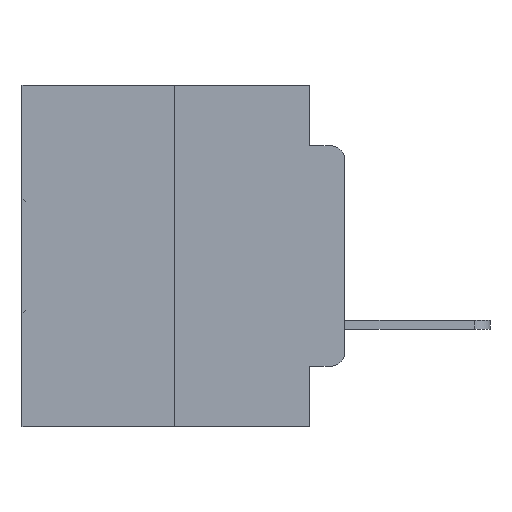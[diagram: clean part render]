
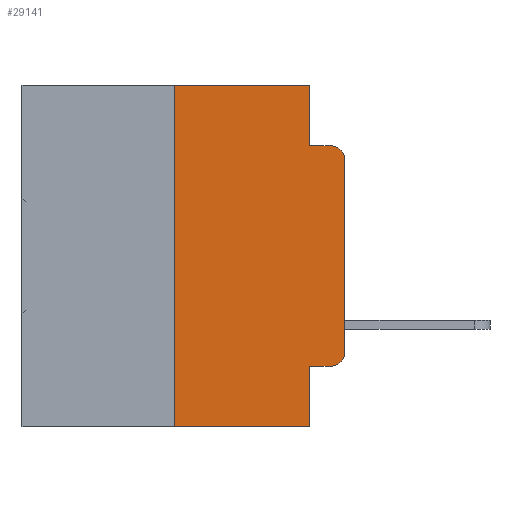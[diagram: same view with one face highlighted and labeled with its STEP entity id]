
A CAD part, left-side view. The second image highlights one B-rep face of the part: STEP entity #29141.
In plain terms, the highlighted planar face has unit normal (-1, 0, 0).
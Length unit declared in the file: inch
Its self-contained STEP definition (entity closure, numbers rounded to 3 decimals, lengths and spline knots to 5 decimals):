
#12 = CARTESIAN_POINT ( 'NONE',  ( 0., 0.25, -0.5 ) ) ;
#432 = EDGE_CURVE ( 'NONE', #4082, #10089, #1228, .T. ) ;
#1228 = CIRCLE ( 'NONE', #27932, 0.02 ) ;
#1529 = AXIS2_PLACEMENT_3D ( 'NONE', #28865, #9449, #2348 ) ;
#2348 = DIRECTION ( 'NONE',  ( 0., 0., -1. ) ) ;
#3346 = DIRECTION ( 'NONE',  ( 0., -1., 0. ) ) ;
#3621 = CARTESIAN_POINT ( 'NONE',  ( 0., 0.051, -0.0885 ) ) ;
#3877 = LINE ( 'NONE', #9337, #23126 ) ;
#4082 = VERTEX_POINT ( 'NONE', #4563 ) ;
#4563 = CARTESIAN_POINT ( 'NONE',  ( 0., 0.02, -0.4115 ) ) ;
#4642 = LINE ( 'NONE', #19260, #14094 ) ;
#4684 = DIRECTION ( 'NONE',  ( 0., 0., -1. ) ) ;
#5099 = ORIENTED_EDGE ( 'NONE', *, *, #18385, .T. ) ;
#5803 = EDGE_CURVE ( 'NONE', #26232, #4082, #29390, .T. ) ;
#7179 = EDGE_CURVE ( 'NONE', #28852, #25640, #28449, .T. ) ;
#8128 = VERTEX_POINT ( 'NONE', #12 ) ;
#8227 = FACE_OUTER_BOUND ( 'NONE', #29650, .T. ) ;
#8229 = DIRECTION ( 'NONE',  ( 0., -1., 0. ) ) ;
#8616 = LINE ( 'NONE', #27436, #13507 ) ;
#8638 = DIRECTION ( 'NONE',  ( 0., 0., -1. ) ) ;
#8962 = VECTOR ( 'NONE', #25877, 39.37008 ) ;
#9337 = CARTESIAN_POINT ( 'NONE',  ( 0., 0.473, -0.5 ) ) ;
#9384 = ORIENTED_EDGE ( 'NONE', *, *, #16188, .F. ) ;
#9449 = DIRECTION ( 'NONE',  ( 1., 0., 0. ) ) ;
#9706 = VECTOR ( 'NONE', #15299, 39.37008 ) ;
#10089 = VERTEX_POINT ( 'NONE', #25922 ) ;
#10110 = CARTESIAN_POINT ( 'NONE',  ( 0., 0.051, 0. ) ) ;
#10231 = VERTEX_POINT ( 'NONE', #29948 ) ;
#10250 = EDGE_CURVE ( 'NONE', #23855, #21568, #8616, .T. ) ;
#10554 = CARTESIAN_POINT ( 'NONE',  ( 0., 0.02, -0.3915 ) ) ;
#11385 = CIRCLE ( 'NONE', #13421, 0.02 ) ;
#11603 = LINE ( 'NONE', #18490, #8962 ) ;
#11885 = ORIENTED_EDGE ( 'NONE', *, *, #10250, .F. ) ;
#12082 = DIRECTION ( 'NONE',  ( 0., 0., 1. ) ) ;
#13181 = DIRECTION ( 'NONE',  ( -1., 0., 0. ) ) ;
#13195 = CARTESIAN_POINT ( 'NONE',  ( 0., 0.25, 0. ) ) ;
#13357 = CARTESIAN_POINT ( 'NONE',  ( 0., 0.25, 0. ) ) ;
#13421 = AXIS2_PLACEMENT_3D ( 'NONE', #21554, #24056, #4684 ) ;
#13507 = VECTOR ( 'NONE', #8229, 39.37008 ) ;
#14094 = VECTOR ( 'NONE', #12082, 39.37008 ) ;
#14629 = ORIENTED_EDGE ( 'NONE', *, *, #5803, .T. ) ;
#15299 = DIRECTION ( 'NONE',  ( 0., 0., 1. ) ) ;
#15474 = CARTESIAN_POINT ( 'NONE',  ( 0., 0.473, 0. ) ) ;
#16108 = LINE ( 'NONE', #13195, #9706 ) ;
#16188 = EDGE_CURVE ( 'NONE', #8128, #28852, #16108, .T. ) ;
#16911 = VERTEX_POINT ( 'NONE', #22786 ) ;
#16942 = CARTESIAN_POINT ( 'NONE',  ( 0., 0.051, -0.4115 ) ) ;
#18385 = EDGE_CURVE ( 'NONE', #8128, #16911, #3877, .T. ) ;
#18438 = ORIENTED_EDGE ( 'NONE', *, *, #26147, .T. ) ;
#18490 = CARTESIAN_POINT ( 'NONE',  ( 0., 0.051, 0. ) ) ;
#18664 = DIRECTION ( 'NONE',  ( 0., -1., 0. ) ) ;
#19215 = LINE ( 'NONE', #20734, #27869 ) ;
#19260 = CARTESIAN_POINT ( 'NONE',  ( 0., 0., 0. ) ) ;
#20734 = CARTESIAN_POINT ( 'NONE',  ( 0., 0.051, 0. ) ) ;
#21186 = CARTESIAN_POINT ( 'NONE',  ( 0., 0.051, -0.4115 ) ) ;
#21554 = CARTESIAN_POINT ( 'NONE',  ( 0., 0.02, -0.1085 ) ) ;
#21568 = VERTEX_POINT ( 'NONE', #29290 ) ;
#21884 = EDGE_CURVE ( 'NONE', #26232, #16911, #11603, .T. ) ;
#22786 = CARTESIAN_POINT ( 'NONE',  ( 0., 0.051, -0.5 ) ) ;
#22878 = ORIENTED_EDGE ( 'NONE', *, *, #27403, .T. ) ;
#23126 = VECTOR ( 'NONE', #26421, 39.37008 ) ;
#23855 = VERTEX_POINT ( 'NONE', #3621 ) ;
#23967 = PLANE ( 'NONE',  #1529 ) ;
#24056 = DIRECTION ( 'NONE',  ( -1., 0., 0. ) ) ;
#24561 = ORIENTED_EDGE ( 'NONE', *, *, #432, .T. ) ;
#25640 = VERTEX_POINT ( 'NONE', #10110 ) ;
#25877 = DIRECTION ( 'NONE',  ( 0., 0., -1. ) ) ;
#25922 = CARTESIAN_POINT ( 'NONE',  ( 0., 0., -0.3915 ) ) ;
#26147 = EDGE_CURVE ( 'NONE', #10089, #10231, #4642, .T. ) ;
#26232 = VERTEX_POINT ( 'NONE', #16942 ) ;
#26421 = DIRECTION ( 'NONE',  ( 0., -1., 0. ) ) ;
#26581 = ORIENTED_EDGE ( 'NONE', *, *, #21884, .F. ) ;
#26897 = VECTOR ( 'NONE', #3346, 39.37008 ) ;
#27403 = EDGE_CURVE ( 'NONE', #10231, #21568, #11385, .T. ) ;
#27436 = CARTESIAN_POINT ( 'NONE',  ( 0., 0.051, -0.0885 ) ) ;
#27494 = VECTOR ( 'NONE', #18664, 39.37008 ) ;
#27869 = VECTOR ( 'NONE', #8638, 39.37008 ) ;
#27932 = AXIS2_PLACEMENT_3D ( 'NONE', #10554, #13181, #29632 ) ;
#28184 = ORIENTED_EDGE ( 'NONE', *, *, #28445, .F. ) ;
#28445 = EDGE_CURVE ( 'NONE', #25640, #23855, #19215, .T. ) ;
#28449 = LINE ( 'NONE', #15474, #26897 ) ;
#28852 = VERTEX_POINT ( 'NONE', #13357 ) ;
#28865 = CARTESIAN_POINT ( 'NONE',  ( 0., 0.473, 0. ) ) ;
#29141 = ADVANCED_FACE ( 'NONE', ( #8227 ), #23967, .F. ) ;
#29290 = CARTESIAN_POINT ( 'NONE',  ( 0., 0.02, -0.0885 ) ) ;
#29390 = LINE ( 'NONE', #21186, #27494 ) ;
#29632 = DIRECTION ( 'NONE',  ( 0., 0., -1. ) ) ;
#29650 = EDGE_LOOP ( 'NONE', ( #18438, #22878, #11885, #28184, #29792, #9384, #5099, #26581, #14629, #24561 ) ) ;
#29792 = ORIENTED_EDGE ( 'NONE', *, *, #7179, .F. ) ;
#29948 = CARTESIAN_POINT ( 'NONE',  ( 0., 0., -0.1085 ) ) ;
